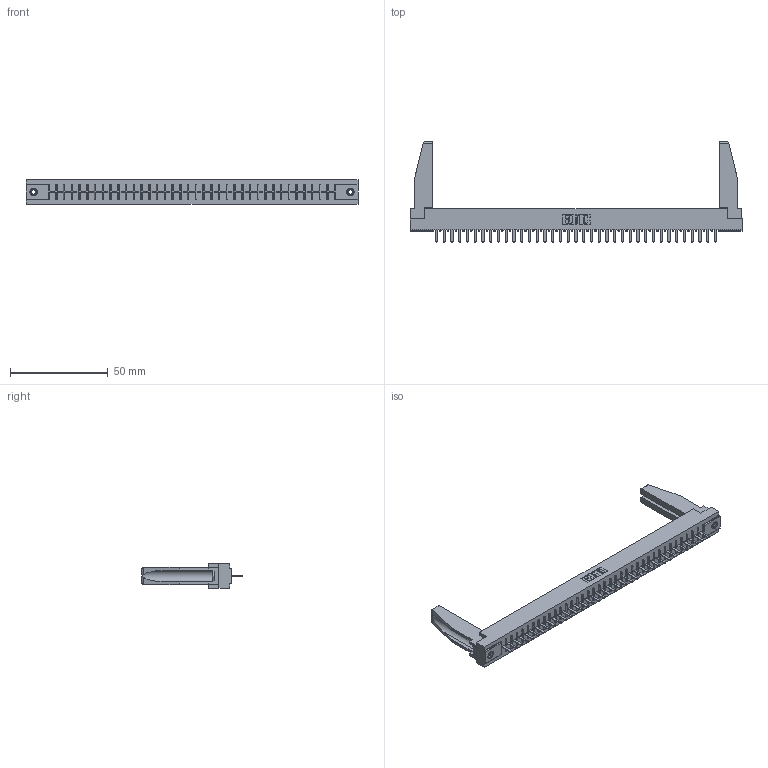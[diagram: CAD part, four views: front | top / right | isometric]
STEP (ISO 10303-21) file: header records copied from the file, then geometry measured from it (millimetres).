
FILE_DESCRIPTION (( 'STEP AP203' ), '1' );
FILE_NAME ('316-037-420-178.STEP', '2020-09-23T05:31:28', ( '' ), ( '' ), 'SwSTEP 2.0', 'SolidWorks 2020', '' );
FILE_SCHEMA (( 'CONFIG_CONTROL_DESIGN' ));
Length unit declared in the file: inch
Products named in the file (5): 306 Part_.156 Dia; 306-290-001_120; 316-037-420-178; 345-250-001_345-250-001-102; 307-220-078
Assembly tree (42 placements, depth 2):
  316-037-420-178
    306 Part_.156 Dia
    306-290-001_120  x37
    345-250-001_345-250-001-102  x2
    307-220-078  x2
Bounding box: 169.62 x 51.16 x 12.7 mm (x, y, z)
Volume: 22718.2 mm3; surface area: 22999.7 mm2
Topology: 42 solids, 42 shells, 2836 faces, 7935 edges, 5082 vertices
Faces by surface type: plane 1891, cylinder 781, sphere 148, cone 12, torus 4
Entity records: 37547 total; most frequent: CARTESIAN_POINT 6304, ORIENTED_EDGE 6208, DIRECTION 6168, EDGE_CURVE 3104, LINE 2428, VECTOR 2428, VERTEX_POINT 1964, AXIS2_PLACEMENT_3D 1870
